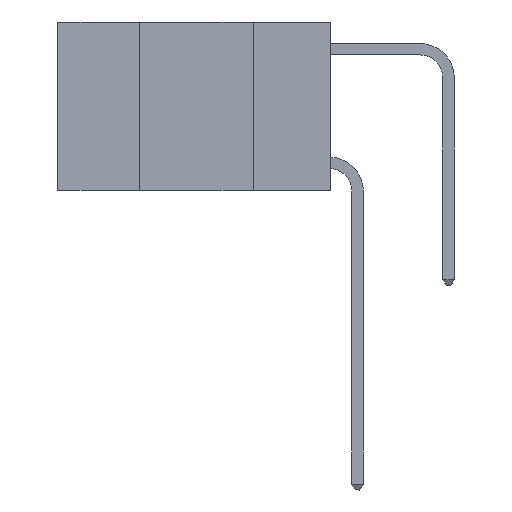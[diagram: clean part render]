
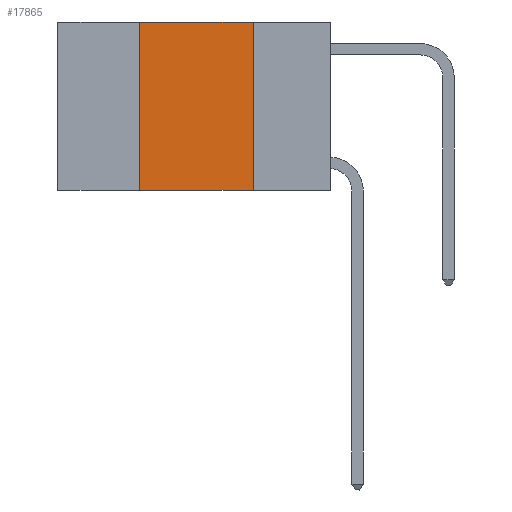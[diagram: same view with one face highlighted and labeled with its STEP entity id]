
A CAD part, left-side view. The second image highlights one B-rep face of the part: STEP entity #17865.
In plain terms, the highlighted planar face has unit normal (-1, 0, 0).
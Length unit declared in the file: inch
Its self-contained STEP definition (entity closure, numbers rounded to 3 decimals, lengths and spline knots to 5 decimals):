
#595 = EDGE_CURVE ( 'NONE', #21709, #1459, #11530, .T. ) ;
#671 = CARTESIAN_POINT ( 'NONE',  ( 0., 0.6, 0. ) ) ;
#1148 = EDGE_CURVE ( 'NONE', #21709, #15123, #25751, .T. ) ;
#1459 = VERTEX_POINT ( 'NONE', #1583 ) ;
#1583 = CARTESIAN_POINT ( 'NONE',  ( 0., 0.42, 0. ) ) ;
#1628 = DIRECTION ( 'NONE',  ( 0., 0., 1. ) ) ;
#2818 = CARTESIAN_POINT ( 'NONE',  ( 0., 0.6, 0. ) ) ;
#4747 = DIRECTION ( 'NONE',  ( 0., 0., -1. ) ) ;
#4879 = FACE_OUTER_BOUND ( 'NONE', #9689, .T. ) ;
#4923 = DIRECTION ( 'NONE',  ( 0., -1., 0. ) ) ;
#5003 = CARTESIAN_POINT ( 'NONE',  ( 0., 0.17, -0.37 ) ) ;
#5207 = LINE ( 'NONE', #2818, #8447 ) ;
#5537 = EDGE_CURVE ( 'NONE', #1459, #17394, #5207, .T. ) ;
#6895 = CARTESIAN_POINT ( 'NONE',  ( 0., 0.17, 0. ) ) ;
#7905 = EDGE_CURVE ( 'NONE', #17394, #15123, #12767, .T. ) ;
#8447 = VECTOR ( 'NONE', #4923, 39.37008 ) ;
#8632 = VECTOR ( 'NONE', #26101, 39.37008 ) ;
#8732 = PLANE ( 'NONE',  #24124 ) ;
#9689 = EDGE_LOOP ( 'NONE', ( #19183, #10970, #13571, #17702 ) ) ;
#10970 = ORIENTED_EDGE ( 'NONE', *, *, #5537, .F. ) ;
#11530 = LINE ( 'NONE', #22532, #20338 ) ;
#12767 = LINE ( 'NONE', #6895, #23172 ) ;
#12843 = DIRECTION ( 'NONE',  ( 1., 0., 0. ) ) ;
#13571 = ORIENTED_EDGE ( 'NONE', *, *, #595, .F. ) ;
#15123 = VERTEX_POINT ( 'NONE', #5003 ) ;
#15600 = CARTESIAN_POINT ( 'NONE',  ( 0., 0.17, 0. ) ) ;
#17394 = VERTEX_POINT ( 'NONE', #15600 ) ;
#17702 = ORIENTED_EDGE ( 'NONE', *, *, #1148, .T. ) ;
#17865 = ADVANCED_FACE ( 'NONE', ( #4879 ), #8732, .F. ) ;
#19183 = ORIENTED_EDGE ( 'NONE', *, *, #7905, .F. ) ;
#20232 = CARTESIAN_POINT ( 'NONE',  ( 0., 0.42, -0.37 ) ) ;
#20338 = VECTOR ( 'NONE', #1628, 39.37008 ) ;
#21709 = VERTEX_POINT ( 'NONE', #20232 ) ;
#22532 = CARTESIAN_POINT ( 'NONE',  ( 0., 0.42, 0. ) ) ;
#23172 = VECTOR ( 'NONE', #25398, 39.37008 ) ;
#24057 = CARTESIAN_POINT ( 'NONE',  ( 0., 0.6, -0.37 ) ) ;
#24124 = AXIS2_PLACEMENT_3D ( 'NONE', #671, #12843, #4747 ) ;
#25398 = DIRECTION ( 'NONE',  ( 0., 0., -1. ) ) ;
#25751 = LINE ( 'NONE', #24057, #8632 ) ;
#26101 = DIRECTION ( 'NONE',  ( 0., -1., 0. ) ) ;
